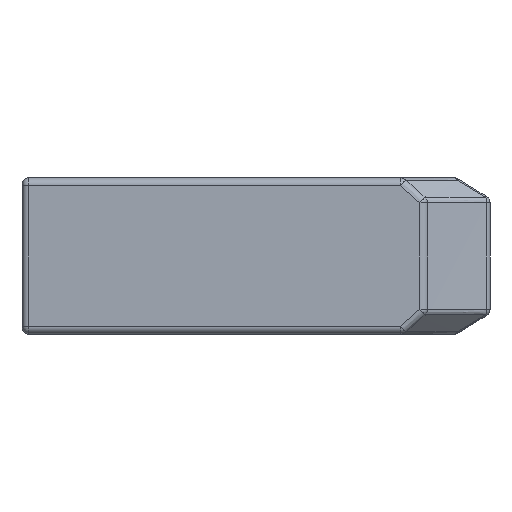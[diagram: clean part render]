
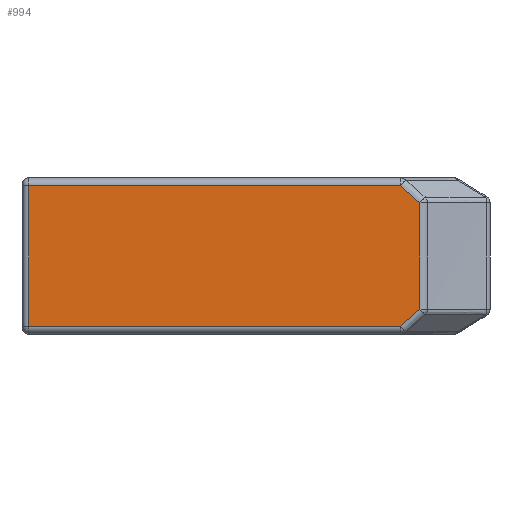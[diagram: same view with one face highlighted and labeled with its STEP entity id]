
A CAD part, front view. The second image highlights one B-rep face of the part: STEP entity #994.
In plain terms, the highlighted planar face has unit normal (0, -1, 0).
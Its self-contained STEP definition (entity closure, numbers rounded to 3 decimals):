
#937=CARTESIAN_POINT('',(-0.5,-11.,33.5));
#938=DIRECTION('',(0.,1.,0.));
#939=DIRECTION('',(-1.,0.,0.));
#940=AXIS2_PLACEMENT_3D('',#937,#938,#939);
#941=PLANE('',#940);
#942=CARTESIAN_POINT('',(6.04,-11.,33.2));
#943=VERTEX_POINT('',#942);
#944=CARTESIAN_POINT('',(-8.25,-11.,33.2));
#945=VERTEX_POINT('',#944);
#946=CARTESIAN_POINT('',(6.04,-11.,33.2));
#947=DIRECTION('',(-1.,0.,-0.));
#948=VECTOR('',#947,14.29);
#949=LINE('',#946,#948);
#950=EDGE_CURVE('',#943,#945,#949,.T.);
#951=ORIENTED_EDGE('',*,*,#950,.T.);
#952=CARTESIAN_POINT('',(-8.25,-11.,27.8));
#953=VERTEX_POINT('',#952);
#954=CARTESIAN_POINT('',(-8.25,-11.,33.2));
#955=DIRECTION('',(0.,0.,-1.));
#956=VECTOR('',#955,5.4);
#957=LINE('',#954,#956);
#958=EDGE_CURVE('',#945,#953,#957,.T.);
#959=ORIENTED_EDGE('',*,*,#958,.T.);
#960=CARTESIAN_POINT('',(6.04,-11.,27.8));
#961=VERTEX_POINT('',#960);
#962=CARTESIAN_POINT('',(-8.25,-11.,27.8));
#963=DIRECTION('',(1.,-0.,0.));
#964=VECTOR('',#963,14.29);
#965=LINE('',#962,#964);
#966=EDGE_CURVE('',#953,#961,#965,.T.);
#967=ORIENTED_EDGE('',*,*,#966,.T.);
#968=CARTESIAN_POINT('',(6.782,-11.,28.458));
#969=VERTEX_POINT('',#968);
#970=CARTESIAN_POINT('',(6.04,-11.,27.8));
#971=CARTESIAN_POINT('',(6.287,-11.,28.02));
#972=CARTESIAN_POINT('',(6.534,-11.,28.239));
#973=CARTESIAN_POINT('',(6.782,-11.,28.458));
#974=B_SPLINE_CURVE_WITH_KNOTS('',3,(#970,#971,#972,#973),.UNSPECIFIED.,.F.,.F.,(4,4),(0.014,0.015),.UNSPECIFIED.);
#975=EDGE_CURVE('',#961,#969,#974,.T.);
#976=ORIENTED_EDGE('',*,*,#975,.T.);
#977=CARTESIAN_POINT('',(6.782,-11.,32.542));
#978=VERTEX_POINT('',#977);
#979=CARTESIAN_POINT('',(6.782,-11.,28.458));
#980=DIRECTION('',(-0.,-0.,1.));
#981=VECTOR('',#980,4.084);
#982=LINE('',#979,#981);
#983=EDGE_CURVE('',#969,#978,#982,.T.);
#984=ORIENTED_EDGE('',*,*,#983,.T.);
#985=CARTESIAN_POINT('',(6.782,-11.,32.542));
#986=CARTESIAN_POINT('',(6.534,-11.,32.761));
#987=CARTESIAN_POINT('',(6.287,-11.,32.98));
#988=CARTESIAN_POINT('',(6.04,-11.,33.2));
#989=B_SPLINE_CURVE_WITH_KNOTS('',3,(#985,#986,#987,#988),.UNSPECIFIED.,.F.,.F.,(4,4),(0.014,0.015),.UNSPECIFIED.);
#990=EDGE_CURVE('',#978,#943,#989,.T.);
#991=ORIENTED_EDGE('',*,*,#990,.T.);
#992=EDGE_LOOP('',(#951,#959,#967,#976,#984,#991));
#993=FACE_BOUND('',#992,.T.);
#994=ADVANCED_FACE('',(#993),#941,.F.);
